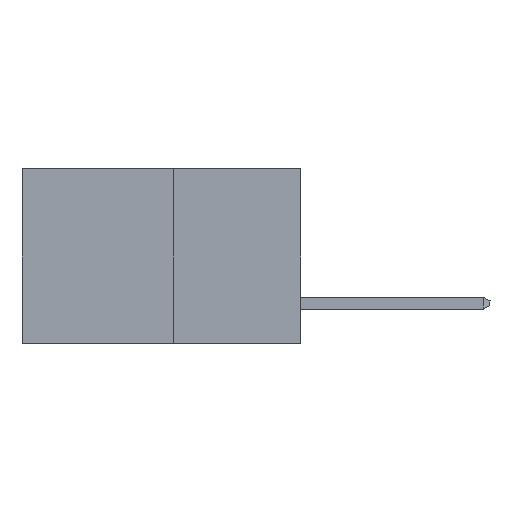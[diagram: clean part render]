
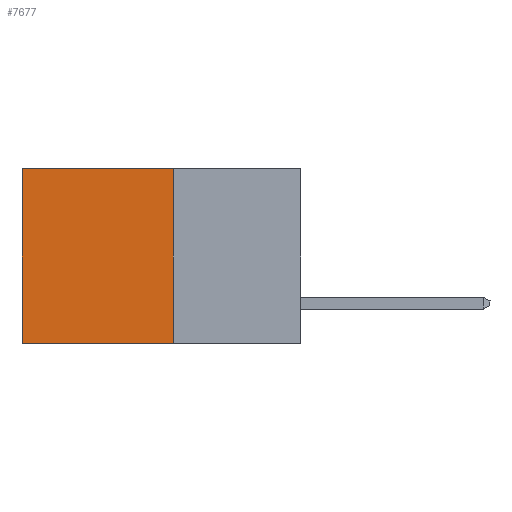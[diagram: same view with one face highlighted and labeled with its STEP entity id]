
A CAD part, left-side view. The second image highlights one B-rep face of the part: STEP entity #7677.
In plain terms, the highlighted planar face has unit normal (-1, 0, 0).
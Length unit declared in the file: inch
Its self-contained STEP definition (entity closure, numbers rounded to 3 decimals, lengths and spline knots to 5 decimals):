
#318 = DIRECTION ( 'NONE',  ( 0., 0., -1. ) ) ;
#338 = CARTESIAN_POINT ( 'NONE',  ( 0.277, 0.27, -0.37 ) ) ;
#351 = ORIENTED_EDGE ( 'NONE', *, *, #4221, .F. ) ;
#1790 = LINE ( 'NONE', #4492, #4114 ) ;
#2126 = EDGE_CURVE ( 'NONE', #4193, #5339, #1790, .T. ) ;
#2240 = CARTESIAN_POINT ( 'NONE',  ( 0.277, 0.27, -0.37 ) ) ;
#2529 = VERTEX_POINT ( 'NONE', #6005 ) ;
#2663 = EDGE_CURVE ( 'NONE', #5339, #2529, #9425, .T. ) ;
#3464 = FACE_OUTER_BOUND ( 'NONE', #9547, .T. ) ;
#3698 = ORIENTED_EDGE ( 'NONE', *, *, #2126, .T. ) ;
#3861 = VERTEX_POINT ( 'NONE', #338 ) ;
#4114 = VECTOR ( 'NONE', #11635, 39.37008 ) ;
#4193 = VERTEX_POINT ( 'NONE', #5986 ) ;
#4221 = EDGE_CURVE ( 'NONE', #3861, #2529, #5267, .T. ) ;
#4492 = CARTESIAN_POINT ( 'NONE',  ( 0.277, 0.27, 0. ) ) ;
#4615 = CARTESIAN_POINT ( 'NONE',  ( 0.277, 0.59, -0.37 ) ) ;
#4732 = VECTOR ( 'NONE', #318, 39.37008 ) ;
#5267 = LINE ( 'NONE', #11136, #11881 ) ;
#5339 = VERTEX_POINT ( 'NONE', #6390 ) ;
#5986 = CARTESIAN_POINT ( 'NONE',  ( 0.277, 0.27, 0. ) ) ;
#6000 = AXIS2_PLACEMENT_3D ( 'NONE', #6521, #6402, #8168 ) ;
#6005 = CARTESIAN_POINT ( 'NONE',  ( 0.277, 0.59, -0.37 ) ) ;
#6390 = CARTESIAN_POINT ( 'NONE',  ( 0.277, 0.59, 0. ) ) ;
#6402 = DIRECTION ( 'NONE',  ( 1., 0., 0. ) ) ;
#6521 = CARTESIAN_POINT ( 'NONE',  ( 0.277, 0.27, -0.37 ) ) ;
#6586 = PLANE ( 'NONE',  #6000 ) ;
#7677 = ADVANCED_FACE ( 'NONE', ( #3464 ), #6586, .F. ) ;
#8168 = DIRECTION ( 'NONE',  ( 0., 0., -1. ) ) ;
#8309 = ORIENTED_EDGE ( 'NONE', *, *, #10966, .F. ) ;
#8701 = DIRECTION ( 'NONE',  ( 0., 0., -1. ) ) ;
#8820 = VECTOR ( 'NONE', #8701, 39.37008 ) ;
#9425 = LINE ( 'NONE', #4615, #4732 ) ;
#9547 = EDGE_LOOP ( 'NONE', ( #11751, #351, #8309, #3698 ) ) ;
#10620 = DIRECTION ( 'NONE',  ( 0., 1., 0. ) ) ;
#10966 = EDGE_CURVE ( 'NONE', #4193, #3861, #11079, .T. ) ;
#11079 = LINE ( 'NONE', #2240, #8820 ) ;
#11136 = CARTESIAN_POINT ( 'NONE',  ( 0.277, 0.27, -0.37 ) ) ;
#11635 = DIRECTION ( 'NONE',  ( 0., 1., 0. ) ) ;
#11751 = ORIENTED_EDGE ( 'NONE', *, *, #2663, .T. ) ;
#11881 = VECTOR ( 'NONE', #10620, 39.37008 ) ;
